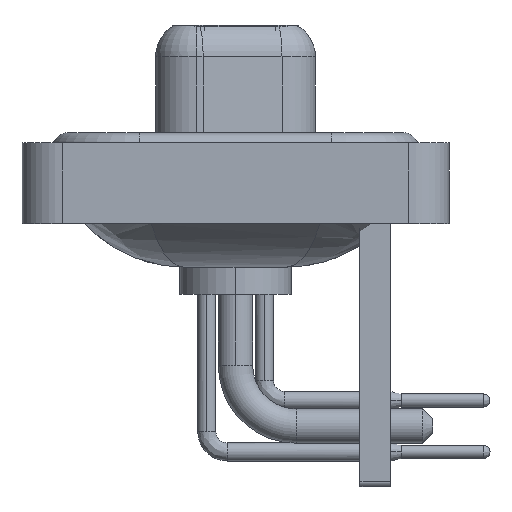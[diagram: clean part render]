
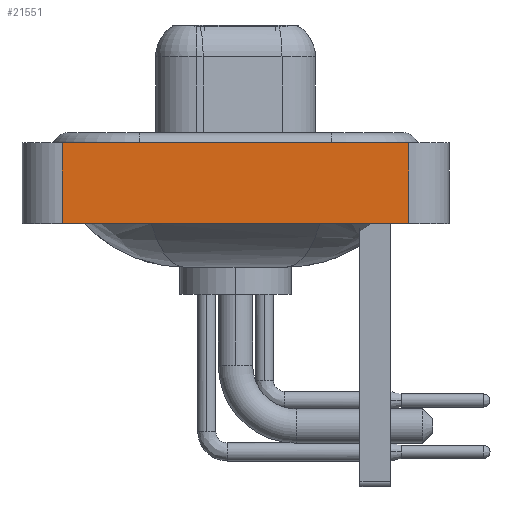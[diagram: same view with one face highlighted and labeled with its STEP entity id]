
A CAD part, left-side view. The second image highlights one B-rep face of the part: STEP entity #21551.
In plain terms, the highlighted planar face has unit normal (-1, 0, 0).
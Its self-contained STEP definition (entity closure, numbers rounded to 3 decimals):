
#150 = DIRECTION ( 'NONE',  ( 0., 0., 1. ) ) ;
#913 = LINE ( 'NONE', #4487, #15677 ) ;
#950 = EDGE_CURVE ( 'NONE', #1315, #17906, #21768, .T. ) ;
#1315 = VERTEX_POINT ( 'NONE', #8930 ) ;
#1942 = PLANE ( 'NONE',  #18320 ) ;
#3539 = CARTESIAN_POINT ( 'NONE',  ( -7.35, -8.55, -3.6 ) ) ;
#4487 = CARTESIAN_POINT ( 'NONE',  ( -7.35, 8.55, -3.6 ) ) ;
#5176 = FACE_OUTER_BOUND ( 'NONE', #10301, .T. ) ;
#5365 = DIRECTION ( 'NONE',  ( 0., 0., 1. ) ) ;
#5455 = DIRECTION ( 'NONE',  ( 0., -1., 0. ) ) ;
#5499 = ORIENTED_EDGE ( 'NONE', *, *, #20648, .F. ) ;
#5733 = VECTOR ( 'NONE', #5365, 1000. ) ;
#7306 = LINE ( 'NONE', #14362, #17000 ) ;
#8388 = VERTEX_POINT ( 'NONE', #20212 ) ;
#8794 = VERTEX_POINT ( 'NONE', #14434 ) ;
#8920 = LINE ( 'NONE', #3539, #18486 ) ;
#8930 = CARTESIAN_POINT ( 'NONE',  ( -7.35, -8.55, -3.6 ) ) ;
#10301 = EDGE_LOOP ( 'NONE', ( #19450, #5499, #21164, #17326 ) ) ;
#12499 = EDGE_CURVE ( 'NONE', #8388, #8794, #913, .T. ) ;
#14362 = CARTESIAN_POINT ( 'NONE',  ( -7.35, -8.55, 0.4 ) ) ;
#14434 = CARTESIAN_POINT ( 'NONE',  ( -7.35, 8.55, 0.4 ) ) ;
#14806 = CARTESIAN_POINT ( 'NONE',  ( -7.35, -8.55, -3.6 ) ) ;
#15633 = DIRECTION ( 'NONE',  ( 0., 0., 1. ) ) ;
#15677 = VECTOR ( 'NONE', #15633, 1000. ) ;
#15897 = EDGE_CURVE ( 'NONE', #8388, #1315, #8920, .T. ) ;
#17000 = VECTOR ( 'NONE', #23614, 1000. ) ;
#17326 = ORIENTED_EDGE ( 'NONE', *, *, #15897, .T. ) ;
#17906 = VERTEX_POINT ( 'NONE', #21298 ) ;
#18121 = CARTESIAN_POINT ( 'NONE',  ( -7.35, -8.55, -3.6 ) ) ;
#18320 = AXIS2_PLACEMENT_3D ( 'NONE', #18121, #20159, #150 ) ;
#18486 = VECTOR ( 'NONE', #5455, 1000. ) ;
#19450 = ORIENTED_EDGE ( 'NONE', *, *, #950, .T. ) ;
#20159 = DIRECTION ( 'NONE',  ( -1., 0., 0. ) ) ;
#20212 = CARTESIAN_POINT ( 'NONE',  ( -7.35, 8.55, -3.6 ) ) ;
#20648 = EDGE_CURVE ( 'NONE', #8794, #17906, #7306, .T. ) ;
#21164 = ORIENTED_EDGE ( 'NONE', *, *, #12499, .F. ) ;
#21298 = CARTESIAN_POINT ( 'NONE',  ( -7.35, -8.55, 0.4 ) ) ;
#21551 = ADVANCED_FACE ( 'NONE', ( #5176 ), #1942, .T. ) ;
#21768 = LINE ( 'NONE', #14806, #5733 ) ;
#23614 = DIRECTION ( 'NONE',  ( 0., -1., 0. ) ) ;
